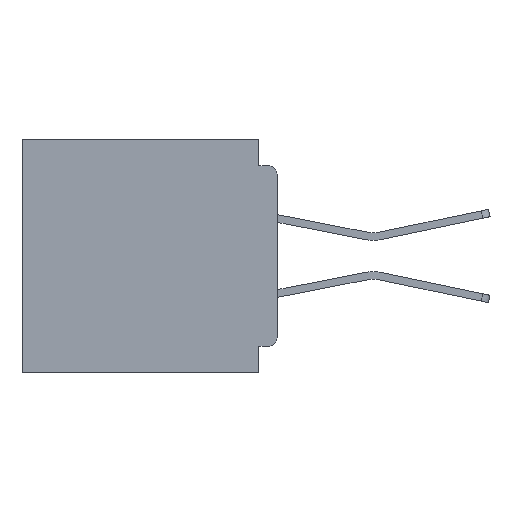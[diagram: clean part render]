
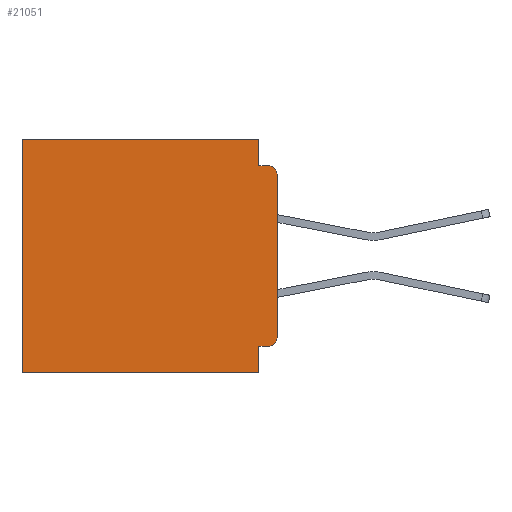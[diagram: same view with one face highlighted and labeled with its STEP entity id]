
A CAD part, left-side view. The second image highlights one B-rep face of the part: STEP entity #21051.
In plain terms, the highlighted planar face has unit normal (-1, 0, 0).
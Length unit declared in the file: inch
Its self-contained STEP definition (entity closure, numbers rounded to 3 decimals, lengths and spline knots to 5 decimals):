
#130 = CARTESIAN_POINT ( 'NONE',  ( 0.3, 0.015, -0.045 ) ) ;
#553 = DIRECTION ( 'NONE',  ( 0., 0., -1. ) ) ;
#740 = DIRECTION ( 'NONE',  ( -1., 0., 0. ) ) ;
#947 = LINE ( 'NONE', #3326, #17734 ) ;
#2287 = ORIENTED_EDGE ( 'NONE', *, *, #18527, .T. ) ;
#2339 = ORIENTED_EDGE ( 'NONE', *, *, #18470, .T. ) ;
#2346 = DIRECTION ( 'NONE',  ( 0., -1., 0. ) ) ;
#3202 = DIRECTION ( 'NONE',  ( 0., 0., -1. ) ) ;
#3326 = CARTESIAN_POINT ( 'NONE',  ( 0.3, 0., -0.4 ) ) ;
#3648 = CIRCLE ( 'NONE', #6749, 0.015 ) ;
#6134 = CARTESIAN_POINT ( 'NONE',  ( 0.3, 0., -0.355 ) ) ;
#6714 = DIRECTION ( 'NONE',  ( 0., 1., 0. ) ) ;
#6749 = AXIS2_PLACEMENT_3D ( 'NONE', #37556, #17703, #40894 ) ;
#6966 = LINE ( 'NONE', #40460, #32456 ) ;
#7382 = DIRECTION ( 'NONE',  ( 0., 1., 0. ) ) ;
#7962 = EDGE_CURVE ( 'NONE', #35103, #16534, #37024, .T. ) ;
#8156 = ORIENTED_EDGE ( 'NONE', *, *, #20451, .F. ) ;
#8660 = CARTESIAN_POINT ( 'NONE',  ( 0.3, 0.031, -0.4 ) ) ;
#8871 = LINE ( 'NONE', #36382, #42099 ) ;
#8970 = CARTESIAN_POINT ( 'NONE',  ( 0.3, 0., -0.045 ) ) ;
#9077 = EDGE_CURVE ( 'NONE', #11110, #32299, #947, .T. ) ;
#9265 = VECTOR ( 'NONE', #9483, 39.37008 ) ;
#9483 = DIRECTION ( 'NONE',  ( 0., 1., 0. ) ) ;
#10615 = EDGE_CURVE ( 'NONE', #39705, #11110, #10883, .T. ) ;
#10883 = LINE ( 'NONE', #8660, #19720 ) ;
#11110 = VERTEX_POINT ( 'NONE', #41275 ) ;
#11168 = CARTESIAN_POINT ( 'NONE',  ( 0.3, 0.437, 0. ) ) ;
#11996 = DIRECTION ( 'NONE',  ( 1., 0., 0. ) ) ;
#13120 = CARTESIAN_POINT ( 'NONE',  ( 0.3, 0., -0.34 ) ) ;
#13936 = LINE ( 'NONE', #8970, #20705 ) ;
#14654 = LINE ( 'NONE', #23964, #31298 ) ;
#15456 = ORIENTED_EDGE ( 'NONE', *, *, #9077, .F. ) ;
#15949 = ORIENTED_EDGE ( 'NONE', *, *, #7962, .T. ) ;
#16463 = FACE_OUTER_BOUND ( 'NONE', #23965, .T. ) ;
#16534 = VERTEX_POINT ( 'NONE', #130 ) ;
#17703 = DIRECTION ( 'NONE',  ( -1., 0., 0. ) ) ;
#17734 = VECTOR ( 'NONE', #6714, 39.37008 ) ;
#17954 = VERTEX_POINT ( 'NONE', #24445 ) ;
#18470 = EDGE_CURVE ( 'NONE', #23029, #37775, #14654, .T. ) ;
#18527 = EDGE_CURVE ( 'NONE', #33115, #21283, #3648, .T. ) ;
#18840 = EDGE_CURVE ( 'NONE', #23029, #17954, #8871, .T. ) ;
#19720 = VECTOR ( 'NONE', #31925, 39.37008 ) ;
#19937 = LINE ( 'NONE', #35213, #27734 ) ;
#20451 = EDGE_CURVE ( 'NONE', #17954, #16534, #13936, .T. ) ;
#20705 = VECTOR ( 'NONE', #2346, 39.37008 ) ;
#20814 = CARTESIAN_POINT ( 'NONE',  ( 0.3, 0.015, -0.06 ) ) ;
#21051 = ADVANCED_FACE ( 'NONE', ( #16463 ), #21906, .F. ) ;
#21283 = VERTEX_POINT ( 'NONE', #13120 ) ;
#21906 = PLANE ( 'NONE',  #22452 ) ;
#22452 = AXIS2_PLACEMENT_3D ( 'NONE', #28555, #11996, #35219 ) ;
#23029 = VERTEX_POINT ( 'NONE', #35125 ) ;
#23262 = ORIENTED_EDGE ( 'NONE', *, *, #23634, .T. ) ;
#23634 = EDGE_CURVE ( 'NONE', #37775, #32299, #19937, .T. ) ;
#23964 = CARTESIAN_POINT ( 'NONE',  ( 0.3, 0., 0. ) ) ;
#23965 = EDGE_LOOP ( 'NONE', ( #32572, #15949, #8156, #36710, #2339, #23262, #15456, #26355, #35190, #2287 ) ) ;
#24149 = DIRECTION ( 'NONE',  ( 0., 0., -1. ) ) ;
#24445 = CARTESIAN_POINT ( 'NONE',  ( 0.3, 0.031, -0.045 ) ) ;
#26355 = ORIENTED_EDGE ( 'NONE', *, *, #10615, .F. ) ;
#27734 = VECTOR ( 'NONE', #38541, 39.37008 ) ;
#28455 = EDGE_CURVE ( 'NONE', #33115, #39705, #35777, .T. ) ;
#28555 = CARTESIAN_POINT ( 'NONE',  ( 0.3, 0., -0.4 ) ) ;
#29111 = CARTESIAN_POINT ( 'NONE',  ( 0.3, 0., -0.06 ) ) ;
#31298 = VECTOR ( 'NONE', #7382, 39.37008 ) ;
#31374 = CARTESIAN_POINT ( 'NONE',  ( 0.3, 0.031, -0.355 ) ) ;
#31925 = DIRECTION ( 'NONE',  ( 0., 0., -1. ) ) ;
#32299 = VERTEX_POINT ( 'NONE', #40094 ) ;
#32456 = VECTOR ( 'NONE', #553, 39.37008 ) ;
#32572 = ORIENTED_EDGE ( 'NONE', *, *, #39669, .F. ) ;
#33115 = VERTEX_POINT ( 'NONE', #41054 ) ;
#35103 = VERTEX_POINT ( 'NONE', #29111 ) ;
#35125 = CARTESIAN_POINT ( 'NONE',  ( 0.3, 0.031, 0. ) ) ;
#35190 = ORIENTED_EDGE ( 'NONE', *, *, #28455, .F. ) ;
#35213 = CARTESIAN_POINT ( 'NONE',  ( 0.3, 0.437, -0.4 ) ) ;
#35219 = DIRECTION ( 'NONE',  ( 0., 0., -1. ) ) ;
#35777 = LINE ( 'NONE', #6134, #9265 ) ;
#36382 = CARTESIAN_POINT ( 'NONE',  ( 0.3, 0.031, 0. ) ) ;
#36710 = ORIENTED_EDGE ( 'NONE', *, *, #18840, .F. ) ;
#37024 = CIRCLE ( 'NONE', #40461, 0.015 ) ;
#37556 = CARTESIAN_POINT ( 'NONE',  ( 0.3, 0.015, -0.34 ) ) ;
#37775 = VERTEX_POINT ( 'NONE', #11168 ) ;
#38541 = DIRECTION ( 'NONE',  ( 0., 0., -1. ) ) ;
#39669 = EDGE_CURVE ( 'NONE', #35103, #21283, #6966, .T. ) ;
#39705 = VERTEX_POINT ( 'NONE', #31374 ) ;
#40094 = CARTESIAN_POINT ( 'NONE',  ( 0.3, 0.437, -0.4 ) ) ;
#40460 = CARTESIAN_POINT ( 'NONE',  ( 0.3, 0., -0.4 ) ) ;
#40461 = AXIS2_PLACEMENT_3D ( 'NONE', #20814, #740, #24149 ) ;
#40894 = DIRECTION ( 'NONE',  ( 0., 0., -1. ) ) ;
#41054 = CARTESIAN_POINT ( 'NONE',  ( 0.3, 0.015, -0.355 ) ) ;
#41275 = CARTESIAN_POINT ( 'NONE',  ( 0.3, 0.031, -0.4 ) ) ;
#42099 = VECTOR ( 'NONE', #3202, 39.37008 ) ;
